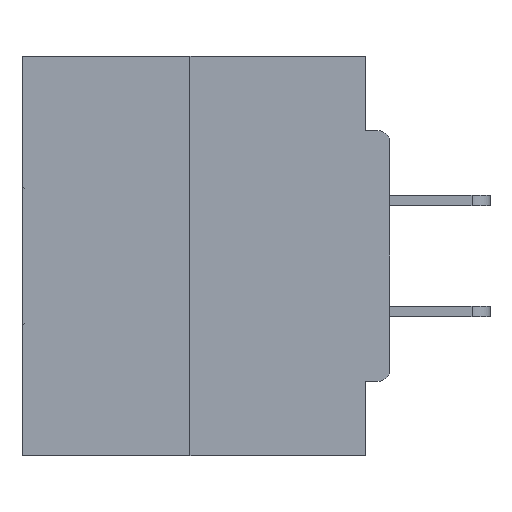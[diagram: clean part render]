
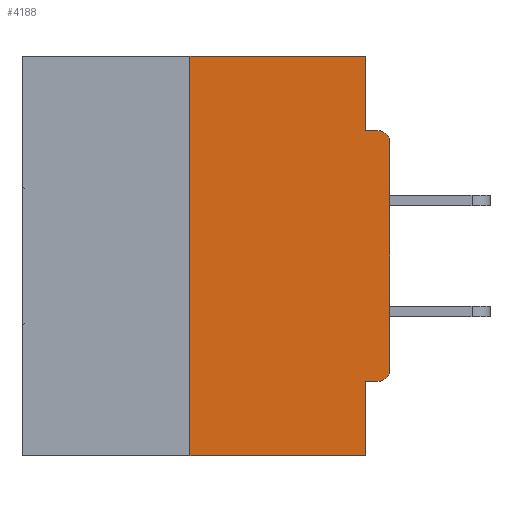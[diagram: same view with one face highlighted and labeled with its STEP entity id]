
A CAD part, left-side view. The second image highlights one B-rep face of the part: STEP entity #4188.
In plain terms, the highlighted planar face has unit normal (-1, 0, 0).
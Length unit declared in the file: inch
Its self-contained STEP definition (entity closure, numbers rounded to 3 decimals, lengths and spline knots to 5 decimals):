
#733 = ORIENTED_EDGE ( 'NONE', *, *, #24293, .F. ) ;
#1215 = CARTESIAN_POINT ( 'NONE',  ( 0., 0.031, -0.0935 ) ) ;
#1871 = CARTESIAN_POINT ( 'NONE',  ( 0., 0.46, 0. ) ) ;
#2192 = ORIENTED_EDGE ( 'NONE', *, *, #29519, .T. ) ;
#2852 = CARTESIAN_POINT ( 'NONE',  ( 0., 0., -0.1085 ) ) ;
#2993 = VERTEX_POINT ( 'NONE', #23092 ) ;
#3423 = LINE ( 'NONE', #6799, #23005 ) ;
#3473 = CARTESIAN_POINT ( 'NONE',  ( 0., 0.25, -0.5 ) ) ;
#3598 = ORIENTED_EDGE ( 'NONE', *, *, #20828, .F. ) ;
#4129 = DIRECTION ( 'NONE',  ( 0., 0., 1. ) ) ;
#4182 = LINE ( 'NONE', #32445, #23726 ) ;
#4188 = ADVANCED_FACE ( 'NONE', ( #11961 ), #38434, .F. ) ;
#4954 = DIRECTION ( 'NONE',  ( 0., 0., -1. ) ) ;
#5264 = VECTOR ( 'NONE', #22828, 39.37008 ) ;
#5824 = LINE ( 'NONE', #24721, #22524 ) ;
#6327 = DIRECTION ( 'NONE',  ( 0., -1., 0. ) ) ;
#6358 = CARTESIAN_POINT ( 'NONE',  ( 0., 0.031, -0.4065 ) ) ;
#6799 = CARTESIAN_POINT ( 'NONE',  ( 0., 0.031, -0.5 ) ) ;
#7207 = CARTESIAN_POINT ( 'NONE',  ( 0., 0.25, 0. ) ) ;
#7960 = CARTESIAN_POINT ( 'NONE',  ( 0., 0.25, 0. ) ) ;
#8438 = LINE ( 'NONE', #32679, #34173 ) ;
#9517 = ORIENTED_EDGE ( 'NONE', *, *, #38366, .F. ) ;
#10501 = EDGE_CURVE ( 'NONE', #13343, #20095, #29614, .T. ) ;
#11663 = CARTESIAN_POINT ( 'NONE',  ( 0., 0.015, -0.0935 ) ) ;
#11758 = ORIENTED_EDGE ( 'NONE', *, *, #26287, .F. ) ;
#11961 = FACE_OUTER_BOUND ( 'NONE', #20756, .T. ) ;
#12299 = DIRECTION ( 'NONE',  ( -1., 0., 0. ) ) ;
#12398 = DIRECTION ( 'NONE',  ( 0., 0., -1. ) ) ;
#12711 = CIRCLE ( 'NONE', #31718, 0.015 ) ;
#13343 = VERTEX_POINT ( 'NONE', #32134 ) ;
#13501 = VERTEX_POINT ( 'NONE', #14366 ) ;
#13772 = CARTESIAN_POINT ( 'NONE',  ( 0., 0.031, 0. ) ) ;
#14157 = ORIENTED_EDGE ( 'NONE', *, *, #17089, .T. ) ;
#14366 = CARTESIAN_POINT ( 'NONE',  ( 0., 0.031, -0.5 ) ) ;
#14510 = CARTESIAN_POINT ( 'NONE',  ( 0., 0.015, -0.3915 ) ) ;
#14764 = VECTOR ( 'NONE', #4129, 39.37008 ) ;
#15110 = DIRECTION ( 'NONE',  ( 0., 0., -1. ) ) ;
#16068 = ORIENTED_EDGE ( 'NONE', *, *, #33047, .T. ) ;
#16421 = ORIENTED_EDGE ( 'NONE', *, *, #24170, .T. ) ;
#16435 = LINE ( 'NONE', #18637, #28828 ) ;
#17089 = EDGE_CURVE ( 'NONE', #33181, #13501, #24720, .T. ) ;
#17464 = DIRECTION ( 'NONE',  ( 0., -1., 0. ) ) ;
#18244 = VERTEX_POINT ( 'NONE', #24541 ) ;
#18637 = CARTESIAN_POINT ( 'NONE',  ( 0., 0.46, 0. ) ) ;
#19927 = DIRECTION ( 'NONE',  ( 1., 0., 0. ) ) ;
#20095 = VERTEX_POINT ( 'NONE', #1215 ) ;
#20756 = EDGE_LOOP ( 'NONE', ( #38138, #3598, #14157, #9517, #11758, #16421, #2192, #16068, #733, #25107 ) ) ;
#20828 = EDGE_CURVE ( 'NONE', #33181, #39315, #28610, .T. ) ;
#20906 = DIRECTION ( 'NONE',  ( -1., 0., 0. ) ) ;
#22524 = VECTOR ( 'NONE', #28061, 39.37008 ) ;
#22828 = DIRECTION ( 'NONE',  ( 0., 0., -1. ) ) ;
#22936 = DIRECTION ( 'NONE',  ( 0., 0., 1. ) ) ;
#23005 = VECTOR ( 'NONE', #12398, 39.37008 ) ;
#23092 = CARTESIAN_POINT ( 'NONE',  ( 0., 0., -0.3915 ) ) ;
#23726 = VECTOR ( 'NONE', #22936, 39.37008 ) ;
#24170 = EDGE_CURVE ( 'NONE', #18244, #2993, #12711, .T. ) ;
#24293 = EDGE_CURVE ( 'NONE', #20095, #26190, #8438, .T. ) ;
#24422 = CARTESIAN_POINT ( 'NONE',  ( 0., 0.015, -0.1085 ) ) ;
#24541 = CARTESIAN_POINT ( 'NONE',  ( 0., 0.015, -0.4065 ) ) ;
#24546 = AXIS2_PLACEMENT_3D ( 'NONE', #1871, #19927, #4954 ) ;
#24720 = LINE ( 'NONE', #30764, #32803 ) ;
#24721 = CARTESIAN_POINT ( 'NONE',  ( 0., 0., -0.4065 ) ) ;
#25107 = ORIENTED_EDGE ( 'NONE', *, *, #10501, .F. ) ;
#25690 = VERTEX_POINT ( 'NONE', #6358 ) ;
#26190 = VERTEX_POINT ( 'NONE', #11663 ) ;
#26287 = EDGE_CURVE ( 'NONE', #18244, #25690, #5824, .T. ) ;
#28061 = DIRECTION ( 'NONE',  ( 0., 1., 0. ) ) ;
#28610 = LINE ( 'NONE', #7207, #14764 ) ;
#28828 = VECTOR ( 'NONE', #6327, 39.37008 ) ;
#29519 = EDGE_CURVE ( 'NONE', #2993, #30437, #4182, .T. ) ;
#29614 = LINE ( 'NONE', #13772, #5264 ) ;
#30437 = VERTEX_POINT ( 'NONE', #2852 ) ;
#30764 = CARTESIAN_POINT ( 'NONE',  ( 0., 0.46, -0.5 ) ) ;
#31615 = CIRCLE ( 'NONE', #36339, 0.015 ) ;
#31718 = AXIS2_PLACEMENT_3D ( 'NONE', #14510, #20906, #39054 ) ;
#32134 = CARTESIAN_POINT ( 'NONE',  ( 0., 0.031, 0. ) ) ;
#32445 = CARTESIAN_POINT ( 'NONE',  ( 0., 0., 0. ) ) ;
#32679 = CARTESIAN_POINT ( 'NONE',  ( 0., 0., -0.0935 ) ) ;
#32803 = VECTOR ( 'NONE', #33716, 39.37008 ) ;
#33047 = EDGE_CURVE ( 'NONE', #30437, #26190, #31615, .T. ) ;
#33181 = VERTEX_POINT ( 'NONE', #3473 ) ;
#33716 = DIRECTION ( 'NONE',  ( 0., -1., 0. ) ) ;
#34173 = VECTOR ( 'NONE', #17464, 39.37008 ) ;
#36339 = AXIS2_PLACEMENT_3D ( 'NONE', #24422, #12299, #15110 ) ;
#37234 = EDGE_CURVE ( 'NONE', #39315, #13343, #16435, .T. ) ;
#38138 = ORIENTED_EDGE ( 'NONE', *, *, #37234, .F. ) ;
#38366 = EDGE_CURVE ( 'NONE', #25690, #13501, #3423, .T. ) ;
#38434 = PLANE ( 'NONE',  #24546 ) ;
#39054 = DIRECTION ( 'NONE',  ( 0., 0., -1. ) ) ;
#39315 = VERTEX_POINT ( 'NONE', #7960 ) ;
